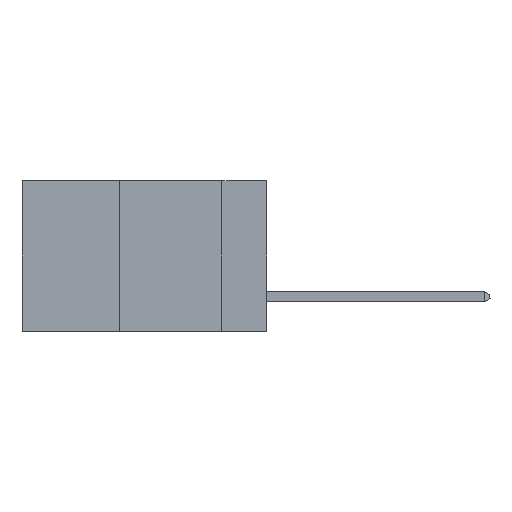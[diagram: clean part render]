
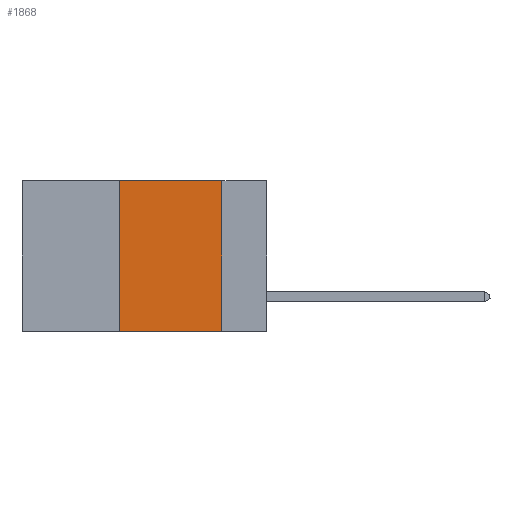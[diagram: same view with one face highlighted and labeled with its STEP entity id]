
A CAD part, left-side view. The second image highlights one B-rep face of the part: STEP entity #1868.
In plain terms, the highlighted planar face has unit normal (-1, 0, 0).
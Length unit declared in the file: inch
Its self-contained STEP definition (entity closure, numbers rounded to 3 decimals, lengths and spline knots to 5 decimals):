
#395 = CARTESIAN_POINT ( 'NONE',  ( 0., 0.6, 0. ) ) ;
#689 = EDGE_CURVE ( 'NONE', #9908, #8971, #2875, .T. ) ;
#703 = PLANE ( 'NONE',  #8919 ) ;
#722 = ORIENTED_EDGE ( 'NONE', *, *, #5037, .F. ) ;
#930 = VECTOR ( 'NONE', #3036, 39.37008 ) ;
#961 = VERTEX_POINT ( 'NONE', #7585 ) ;
#1472 = CARTESIAN_POINT ( 'NONE',  ( 0., 0.6, 0. ) ) ;
#1579 = EDGE_CURVE ( 'NONE', #961, #9908, #9730, .T. ) ;
#1850 = ORIENTED_EDGE ( 'NONE', *, *, #689, .F. ) ;
#1868 = ADVANCED_FACE ( 'NONE', ( #2469 ), #703, .F. ) ;
#1889 = CARTESIAN_POINT ( 'NONE',  ( 0., 0.36, -0.37 ) ) ;
#2056 = DIRECTION ( 'NONE',  ( 0., -1., 0. ) ) ;
#2469 = FACE_OUTER_BOUND ( 'NONE', #3692, .T. ) ;
#2875 = LINE ( 'NONE', #10412, #930 ) ;
#3036 = DIRECTION ( 'NONE',  ( 0., 0., -1. ) ) ;
#3191 = VERTEX_POINT ( 'NONE', #1889 ) ;
#3692 = EDGE_LOOP ( 'NONE', ( #1850, #10484, #722, #9780 ) ) ;
#3874 = CARTESIAN_POINT ( 'NONE',  ( 0., 0.11, 0. ) ) ;
#3923 = DIRECTION ( 'NONE',  ( 0., 0., -1. ) ) ;
#4942 = DIRECTION ( 'NONE',  ( 0., 0., 1. ) ) ;
#5037 = EDGE_CURVE ( 'NONE', #3191, #961, #6622, .T. ) ;
#5245 = DIRECTION ( 'NONE',  ( 0., -1., 0. ) ) ;
#5597 = DIRECTION ( 'NONE',  ( 1., 0., 0. ) ) ;
#6622 = LINE ( 'NONE', #7183, #8691 ) ;
#7183 = CARTESIAN_POINT ( 'NONE',  ( 0., 0.36, 0. ) ) ;
#7521 = VECTOR ( 'NONE', #2056, 39.37008 ) ;
#7585 = CARTESIAN_POINT ( 'NONE',  ( 0., 0.36, 0. ) ) ;
#8206 = VECTOR ( 'NONE', #5245, 39.37008 ) ;
#8227 = CARTESIAN_POINT ( 'NONE',  ( 0., 0.11, -0.37 ) ) ;
#8691 = VECTOR ( 'NONE', #4942, 39.37008 ) ;
#8919 = AXIS2_PLACEMENT_3D ( 'NONE', #1472, #5597, #3923 ) ;
#8971 = VERTEX_POINT ( 'NONE', #8227 ) ;
#9223 = LINE ( 'NONE', #10284, #8206 ) ;
#9730 = LINE ( 'NONE', #395, #7521 ) ;
#9780 = ORIENTED_EDGE ( 'NONE', *, *, #10344, .T. ) ;
#9908 = VERTEX_POINT ( 'NONE', #3874 ) ;
#10284 = CARTESIAN_POINT ( 'NONE',  ( 0., 0.6, -0.37 ) ) ;
#10344 = EDGE_CURVE ( 'NONE', #3191, #8971, #9223, .T. ) ;
#10412 = CARTESIAN_POINT ( 'NONE',  ( 0., 0.11, 0. ) ) ;
#10484 = ORIENTED_EDGE ( 'NONE', *, *, #1579, .F. ) ;
